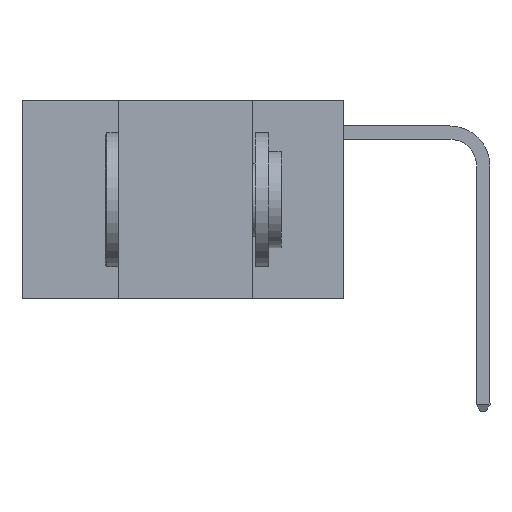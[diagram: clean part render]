
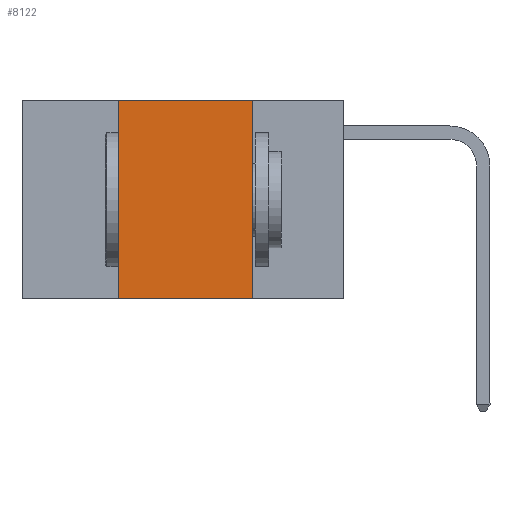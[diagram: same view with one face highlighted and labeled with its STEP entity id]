
A CAD part, left-side view. The second image highlights one B-rep face of the part: STEP entity #8122.
In plain terms, the highlighted planar face has unit normal (-1, 0, 0).
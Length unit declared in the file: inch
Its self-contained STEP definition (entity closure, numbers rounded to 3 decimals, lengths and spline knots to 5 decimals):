
#214 = EDGE_CURVE ( 'NONE', #3272, #2834, #10738, .T. ) ;
#852 = VECTOR ( 'NONE', #10470, 39.37008 ) ;
#1743 = ORIENTED_EDGE ( 'NONE', *, *, #10171, .F. ) ;
#1753 = ORIENTED_EDGE ( 'NONE', *, *, #3506, .F. ) ;
#1764 = ORIENTED_EDGE ( 'NONE', *, *, #6737, .F. ) ;
#1789 = ORIENTED_EDGE ( 'NONE', *, *, #214, .T. ) ;
#1981 = AXIS2_PLACEMENT_3D ( 'NONE', #3584, #4380, #4161 ) ;
#2717 = VERTEX_POINT ( 'NONE', #10112 ) ;
#2834 = VERTEX_POINT ( 'NONE', #10495 ) ;
#3013 = CARTESIAN_POINT ( 'NONE',  ( 0., 0.17, 0. ) ) ;
#3272 = VERTEX_POINT ( 'NONE', #10348 ) ;
#3462 = DIRECTION ( 'NONE',  ( 0., -1., 0. ) ) ;
#3506 = EDGE_CURVE ( 'NONE', #2717, #7190, #10852, .T. ) ;
#3584 = CARTESIAN_POINT ( 'NONE',  ( 0., 0.6, 0. ) ) ;
#3699 = DIRECTION ( 'NONE',  ( 0., -1., 0. ) ) ;
#3772 = CARTESIAN_POINT ( 'NONE',  ( 0., 0.6, 0. ) ) ;
#4161 = DIRECTION ( 'NONE',  ( 0., 0., -1. ) ) ;
#4235 = FACE_OUTER_BOUND ( 'NONE', #4689, .T. ) ;
#4267 = VECTOR ( 'NONE', #3462, 39.37008 ) ;
#4380 = DIRECTION ( 'NONE',  ( 1., 0., 0. ) ) ;
#4689 = EDGE_LOOP ( 'NONE', ( #1743, #1753, #1764, #1789 ) ) ;
#5342 = PLANE ( 'NONE',  #1981 ) ;
#5890 = CARTESIAN_POINT ( 'NONE',  ( 0., 0.17, 0. ) ) ;
#6159 = CARTESIAN_POINT ( 'NONE',  ( 0., 0.6, -0.37 ) ) ;
#6737 = EDGE_CURVE ( 'NONE', #3272, #2717, #7616, .T. ) ;
#7190 = VERTEX_POINT ( 'NONE', #5890 ) ;
#7584 = LINE ( 'NONE', #3013, #852 ) ;
#7595 = VECTOR ( 'NONE', #9748, 39.37008 ) ;
#7616 = LINE ( 'NONE', #9857, #7595 ) ;
#8122 = ADVANCED_FACE ( 'NONE', ( #4235 ), #5342, .F. ) ;
#9748 = DIRECTION ( 'NONE',  ( 0., 0., 1. ) ) ;
#9857 = CARTESIAN_POINT ( 'NONE',  ( 0., 0.42, 0. ) ) ;
#10112 = CARTESIAN_POINT ( 'NONE',  ( 0., 0.42, 0. ) ) ;
#10171 = EDGE_CURVE ( 'NONE', #7190, #2834, #7584, .T. ) ;
#10348 = CARTESIAN_POINT ( 'NONE',  ( 0., 0.42, -0.37 ) ) ;
#10470 = DIRECTION ( 'NONE',  ( 0., 0., -1. ) ) ;
#10495 = CARTESIAN_POINT ( 'NONE',  ( 0., 0.17, -0.37 ) ) ;
#10738 = LINE ( 'NONE', #6159, #10772 ) ;
#10772 = VECTOR ( 'NONE', #3699, 39.37008 ) ;
#10852 = LINE ( 'NONE', #3772, #4267 ) ;
